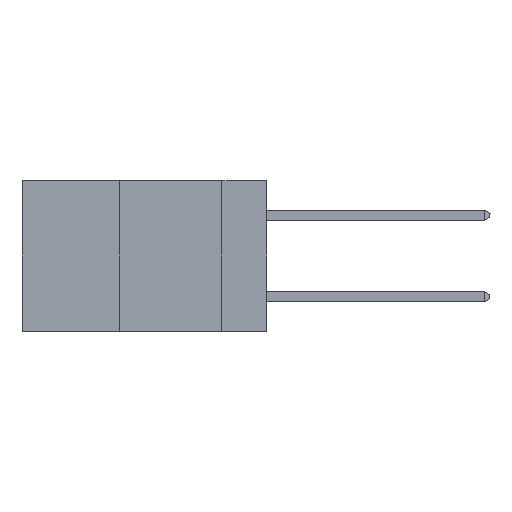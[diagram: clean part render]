
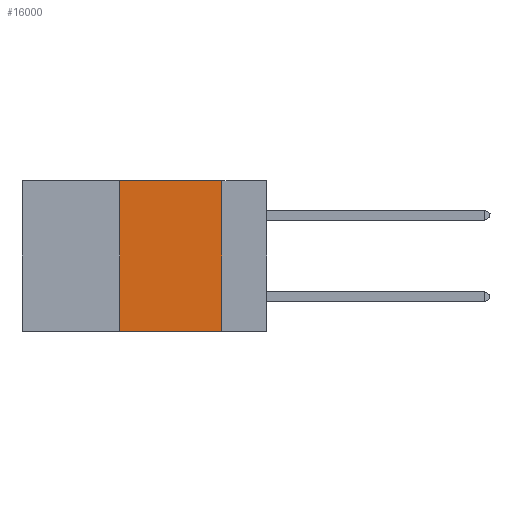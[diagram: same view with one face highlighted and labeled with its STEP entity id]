
A CAD part, left-side view. The second image highlights one B-rep face of the part: STEP entity #16000.
In plain terms, the highlighted planar face has unit normal (-1, 0, 0).
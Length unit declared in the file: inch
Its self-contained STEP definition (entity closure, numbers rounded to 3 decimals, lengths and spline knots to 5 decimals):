
#208 = CARTESIAN_POINT ( 'NONE',  ( 0., 0.11, 0. ) ) ;
#394 = ORIENTED_EDGE ( 'NONE', *, *, #17439, .F. ) ;
#1047 = DIRECTION ( 'NONE',  ( 0., 0., 1. ) ) ;
#1688 = LINE ( 'NONE', #20259, #19359 ) ;
#1956 = CARTESIAN_POINT ( 'NONE',  ( 0., 0.6, -0.37 ) ) ;
#2304 = DIRECTION ( 'NONE',  ( 0., 0., -1. ) ) ;
#4487 = VECTOR ( 'NONE', #1047, 39.37008 ) ;
#5038 = LINE ( 'NONE', #21439, #4487 ) ;
#5874 = EDGE_CURVE ( 'NONE', #13087, #17963, #11960, .T. ) ;
#7288 = DIRECTION ( 'NONE',  ( 0., -1., 0. ) ) ;
#7561 = CARTESIAN_POINT ( 'NONE',  ( 0., 0.6, 0. ) ) ;
#8643 = FACE_OUTER_BOUND ( 'NONE', #21785, .T. ) ;
#9286 = DIRECTION ( 'NONE',  ( 1., 0., 0. ) ) ;
#9829 = CARTESIAN_POINT ( 'NONE',  ( 0., 0.11, -0.37 ) ) ;
#10159 = DIRECTION ( 'NONE',  ( 0., -1., 0. ) ) ;
#10917 = CARTESIAN_POINT ( 'NONE',  ( 0., 0.36, -0.37 ) ) ;
#11085 = EDGE_CURVE ( 'NONE', #11632, #17963, #16201, .T. ) ;
#11632 = VERTEX_POINT ( 'NONE', #208 ) ;
#11960 = LINE ( 'NONE', #1956, #20293 ) ;
#12656 = PLANE ( 'NONE',  #20742 ) ;
#12696 = ORIENTED_EDGE ( 'NONE', *, *, #5874, .T. ) ;
#13087 = VERTEX_POINT ( 'NONE', #10917 ) ;
#14494 = CARTESIAN_POINT ( 'NONE',  ( 0., 0.36, 0. ) ) ;
#15722 = ORIENTED_EDGE ( 'NONE', *, *, #17281, .F. ) ;
#16000 = ADVANCED_FACE ( 'NONE', ( #8643 ), #12656, .F. ) ;
#16041 = VERTEX_POINT ( 'NONE', #14494 ) ;
#16201 = LINE ( 'NONE', #20961, #17769 ) ;
#17281 = EDGE_CURVE ( 'NONE', #13087, #16041, #5038, .T. ) ;
#17439 = EDGE_CURVE ( 'NONE', #16041, #11632, #1688, .T. ) ;
#17769 = VECTOR ( 'NONE', #2304, 39.37008 ) ;
#17963 = VERTEX_POINT ( 'NONE', #9829 ) ;
#18417 = ORIENTED_EDGE ( 'NONE', *, *, #11085, .F. ) ;
#19359 = VECTOR ( 'NONE', #10159, 39.37008 ) ;
#20259 = CARTESIAN_POINT ( 'NONE',  ( 0., 0.6, 0. ) ) ;
#20293 = VECTOR ( 'NONE', #7288, 39.37008 ) ;
#20742 = AXIS2_PLACEMENT_3D ( 'NONE', #7561, #9286, #20980 ) ;
#20961 = CARTESIAN_POINT ( 'NONE',  ( 0., 0.11, 0. ) ) ;
#20980 = DIRECTION ( 'NONE',  ( 0., 0., -1. ) ) ;
#21439 = CARTESIAN_POINT ( 'NONE',  ( 0., 0.36, 0. ) ) ;
#21785 = EDGE_LOOP ( 'NONE', ( #18417, #394, #15722, #12696 ) ) ;
